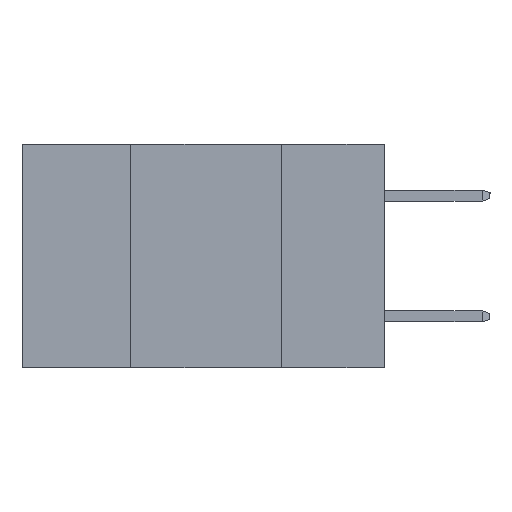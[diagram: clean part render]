
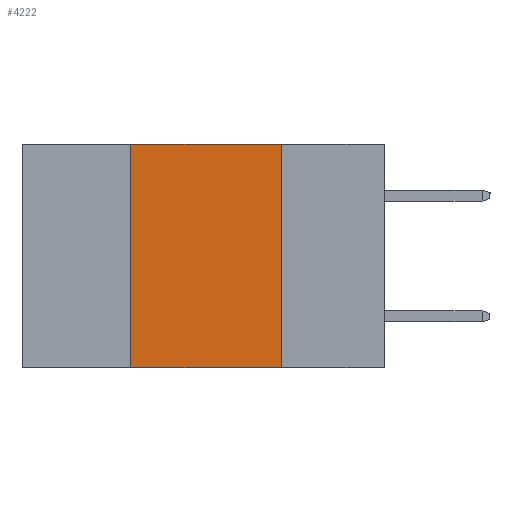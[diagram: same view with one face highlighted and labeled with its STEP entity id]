
A CAD part, left-side view. The second image highlights one B-rep face of the part: STEP entity #4222.
In plain terms, the highlighted planar face has unit normal (-1, 0, 0).
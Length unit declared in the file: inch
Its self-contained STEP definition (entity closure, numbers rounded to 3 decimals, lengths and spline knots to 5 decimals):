
#149 = VERTEX_POINT ( 'NONE', #5535 ) ;
#236 = LINE ( 'NONE', #5220, #6354 ) ;
#490 = EDGE_CURVE ( 'NONE', #3794, #6263, #236, .T. ) ;
#576 = CARTESIAN_POINT ( 'NONE',  ( 0., 0.42, -0.37 ) ) ;
#715 = VECTOR ( 'NONE', #3488, 39.37008 ) ;
#723 = VECTOR ( 'NONE', #3900, 39.37008 ) ;
#1194 = EDGE_LOOP ( 'NONE', ( #1807, #3241, #4386, #2870 ) ) ;
#1365 = CARTESIAN_POINT ( 'NONE',  ( 0., 0.6, 0. ) ) ;
#1411 = DIRECTION ( 'NONE',  ( 1., 0., 0. ) ) ;
#1542 = CARTESIAN_POINT ( 'NONE',  ( 0., 0.6, 0. ) ) ;
#1807 = ORIENTED_EDGE ( 'NONE', *, *, #490, .F. ) ;
#1995 = VECTOR ( 'NONE', #4241, 39.37008 ) ;
#2870 = ORIENTED_EDGE ( 'NONE', *, *, #3119, .T. ) ;
#2963 = EDGE_CURVE ( 'NONE', #2972, #3794, #3761, .T. ) ;
#2972 = VERTEX_POINT ( 'NONE', #3715 ) ;
#3095 = CARTESIAN_POINT ( 'NONE',  ( 0., 0.6, -0.37 ) ) ;
#3119 = EDGE_CURVE ( 'NONE', #149, #6263, #4671, .T. ) ;
#3241 = ORIENTED_EDGE ( 'NONE', *, *, #2963, .F. ) ;
#3488 = DIRECTION ( 'NONE',  ( 0., -1., 0. ) ) ;
#3509 = AXIS2_PLACEMENT_3D ( 'NONE', #1365, #1411, #8554 ) ;
#3715 = CARTESIAN_POINT ( 'NONE',  ( 0., 0.42, 0. ) ) ;
#3761 = LINE ( 'NONE', #1542, #715 ) ;
#3794 = VERTEX_POINT ( 'NONE', #7161 ) ;
#3900 = DIRECTION ( 'NONE',  ( 0., -1., 0. ) ) ;
#4222 = ADVANCED_FACE ( 'NONE', ( #4381 ), #6301, .F. ) ;
#4241 = DIRECTION ( 'NONE',  ( 0., 0., 1. ) ) ;
#4381 = FACE_OUTER_BOUND ( 'NONE', #1194, .T. ) ;
#4386 = ORIENTED_EDGE ( 'NONE', *, *, #4692, .F. ) ;
#4671 = LINE ( 'NONE', #3095, #723 ) ;
#4692 = EDGE_CURVE ( 'NONE', #149, #2972, #4958, .T. ) ;
#4958 = LINE ( 'NONE', #576, #1995 ) ;
#5220 = CARTESIAN_POINT ( 'NONE',  ( 0., 0.17, -0.37 ) ) ;
#5327 = CARTESIAN_POINT ( 'NONE',  ( 0., 0.17, -0.37 ) ) ;
#5535 = CARTESIAN_POINT ( 'NONE',  ( 0., 0.42, -0.37 ) ) ;
#6263 = VERTEX_POINT ( 'NONE', #5327 ) ;
#6301 = PLANE ( 'NONE',  #3509 ) ;
#6354 = VECTOR ( 'NONE', #8767, 39.37008 ) ;
#7161 = CARTESIAN_POINT ( 'NONE',  ( 0., 0.17, 0. ) ) ;
#8554 = DIRECTION ( 'NONE',  ( 0., 0., -1. ) ) ;
#8767 = DIRECTION ( 'NONE',  ( 0., 0., -1. ) ) ;
